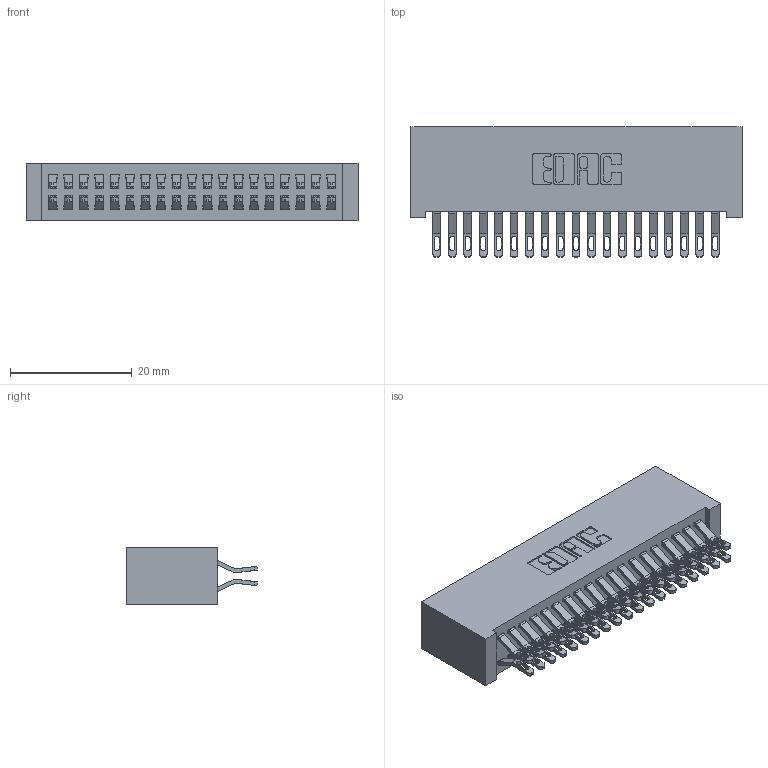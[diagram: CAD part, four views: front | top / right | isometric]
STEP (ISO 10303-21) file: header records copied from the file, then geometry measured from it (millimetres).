
FILE_DESCRIPTION (( 'STEP AP203' ), '1' );
FILE_NAME ('342-038-555-201.STEP', '2019-10-02T14:59:59', ( '' ), ( '' ), 'SwSTEP 2.0', 'SolidWorks 2016', '' );
FILE_SCHEMA (( 'CONFIG_CONTROL_DESIGN' ));
Length unit declared in the file: inch
Products named in the file (3): 342 Part_Lugless; 345-292-001_555 Tail; 342-038-555-201
Assembly tree (39 placements, depth 2):
  342-038-555-201
    342 Part_Lugless
    345-292-001_555 Tail  x38
Bounding box: 54.51 x 21.47 x 9.4 mm (x, y, z)
Volume: 5333.8 mm3; surface area: 8929.3 mm2
Topology: 39 solids, 39 shells, 2306 faces, 7229 edges, 4818 vertices
Faces by surface type: plane 1354, cylinder 952
Entity records: 15115 total; most frequent: CARTESIAN_POINT 2564, ORIENTED_EDGE 2470, DIRECTION 2195, EDGE_CURVE 1235, LINE 1095, VECTOR 1095, VERTEX_POINT 822, AXIS2_PLACEMENT_3D 550
